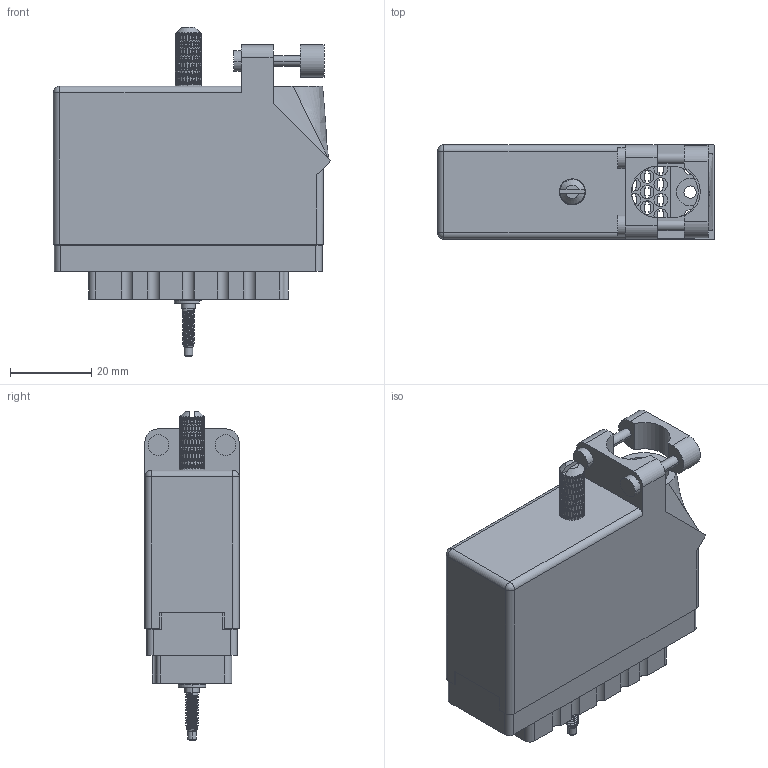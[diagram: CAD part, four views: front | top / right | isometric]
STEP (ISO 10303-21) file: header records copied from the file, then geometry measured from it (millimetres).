
FILE_DESCRIPTION (( 'STEP AP203' ), '1' );
FILE_NAME ('516-056-000-615.STEP', '2020-03-05T20:34:59', ( '' ), ( '' ), 'SwSTEP 2.0', 'SolidWorks 2016', '' );
FILE_SCHEMA (( 'CONFIG_CONTROL_DESIGN' ));
Length unit declared in the file: inch
Products named in the file (8): 516-230-001_Plastic - 056 Top Entry; 516-250-038-111; 516-253-035-100; 516-056-000-615; 516-253-138-107; 516-251-035-100; Actuating Screw Assy 038-056; 516 Part Receptacle_056
Assembly tree (8 placements, depth 3):
  516-056-000-615
    516 Part Receptacle_056
    516-230-001_Plastic - 056 Top Entry
    Actuating Screw Assy 038-056
      516-251-035-100
      516-253-035-100  x2
      516-253-138-107
      516-250-038-111
Bounding box: 68.14 x 23.11 x 81.03 mm (x, y, z)
Volume: 28561.1 mm3; surface area: 38827 mm2
Topology: 7 solids, 7 shells, 2737 faces, 6928 edges, 4228 vertices
Faces by surface type: bspline 1009, plane 1006, cylinder 700, cone 20, sphere 2
Entity records: 111910 total; most frequent: CARTESIAN_POINT 56133, ORIENTED_EDGE 13828, DIRECTION 8926, EDGE_CURVE 6914, VERTEX_POINT 4220, LINE 3016, VECTOR 3016, AXIS2_PLACEMENT_3D 2955
